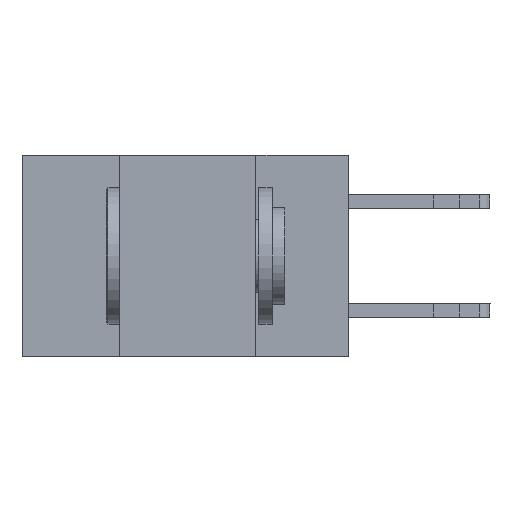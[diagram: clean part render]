
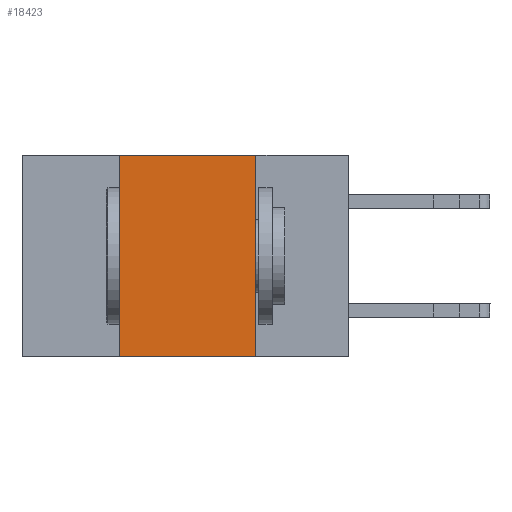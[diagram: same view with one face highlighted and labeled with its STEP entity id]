
A CAD part, left-side view. The second image highlights one B-rep face of the part: STEP entity #18423.
In plain terms, the highlighted planar face has unit normal (-1, 0, 0).
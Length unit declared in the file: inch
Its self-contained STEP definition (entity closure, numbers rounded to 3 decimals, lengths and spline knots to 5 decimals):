
#652 = VECTOR ( 'NONE', #3660, 39.37008 ) ;
#1402 = EDGE_LOOP ( 'NONE', ( #14632, #14812, #18772, #20437 ) ) ;
#1589 = CARTESIAN_POINT ( 'NONE',  ( 0., 0.6, -0.37 ) ) ;
#2540 = AXIS2_PLACEMENT_3D ( 'NONE', #13468, #11582, #21202 ) ;
#3660 = DIRECTION ( 'NONE',  ( 0., -1., 0. ) ) ;
#3794 = EDGE_CURVE ( 'NONE', #20992, #24386, #9609, .T. ) ;
#4712 = CARTESIAN_POINT ( 'NONE',  ( 0., 0.17, -0.37 ) ) ;
#5692 = DIRECTION ( 'NONE',  ( 0., -1., 0. ) ) ;
#5849 = CARTESIAN_POINT ( 'NONE',  ( 0., 0.42, -0.37 ) ) ;
#5891 = FACE_OUTER_BOUND ( 'NONE', #1402, .T. ) ;
#6708 = LINE ( 'NONE', #17356, #24844 ) ;
#7575 = EDGE_CURVE ( 'NONE', #12030, #18818, #9734, .T. ) ;
#9609 = LINE ( 'NONE', #11192, #12741 ) ;
#9734 = LINE ( 'NONE', #22561, #15636 ) ;
#11032 = DIRECTION ( 'NONE',  ( 0., 0., -1. ) ) ;
#11192 = CARTESIAN_POINT ( 'NONE',  ( 0., 0.17, 0. ) ) ;
#11315 = LINE ( 'NONE', #1589, #652 ) ;
#11582 = DIRECTION ( 'NONE',  ( 1., 0., 0. ) ) ;
#12030 = VERTEX_POINT ( 'NONE', #5849 ) ;
#12741 = VECTOR ( 'NONE', #11032, 39.37008 ) ;
#13468 = CARTESIAN_POINT ( 'NONE',  ( 0., 0.6, 0. ) ) ;
#14632 = ORIENTED_EDGE ( 'NONE', *, *, #3794, .F. ) ;
#14812 = ORIENTED_EDGE ( 'NONE', *, *, #23269, .F. ) ;
#15636 = VECTOR ( 'NONE', #16652, 39.37008 ) ;
#16652 = DIRECTION ( 'NONE',  ( 0., 0., 1. ) ) ;
#16752 = CARTESIAN_POINT ( 'NONE',  ( 0., 0.17, 0. ) ) ;
#17356 = CARTESIAN_POINT ( 'NONE',  ( 0., 0.6, 0. ) ) ;
#18423 = ADVANCED_FACE ( 'NONE', ( #5891 ), #21122, .F. ) ;
#18772 = ORIENTED_EDGE ( 'NONE', *, *, #7575, .F. ) ;
#18818 = VERTEX_POINT ( 'NONE', #24413 ) ;
#20437 = ORIENTED_EDGE ( 'NONE', *, *, #20672, .T. ) ;
#20672 = EDGE_CURVE ( 'NONE', #12030, #24386, #11315, .T. ) ;
#20992 = VERTEX_POINT ( 'NONE', #16752 ) ;
#21122 = PLANE ( 'NONE',  #2540 ) ;
#21202 = DIRECTION ( 'NONE',  ( 0., 0., -1. ) ) ;
#22561 = CARTESIAN_POINT ( 'NONE',  ( 0., 0.42, 0. ) ) ;
#23269 = EDGE_CURVE ( 'NONE', #18818, #20992, #6708, .T. ) ;
#24386 = VERTEX_POINT ( 'NONE', #4712 ) ;
#24413 = CARTESIAN_POINT ( 'NONE',  ( 0., 0.42, 0. ) ) ;
#24844 = VECTOR ( 'NONE', #5692, 39.37008 ) ;
